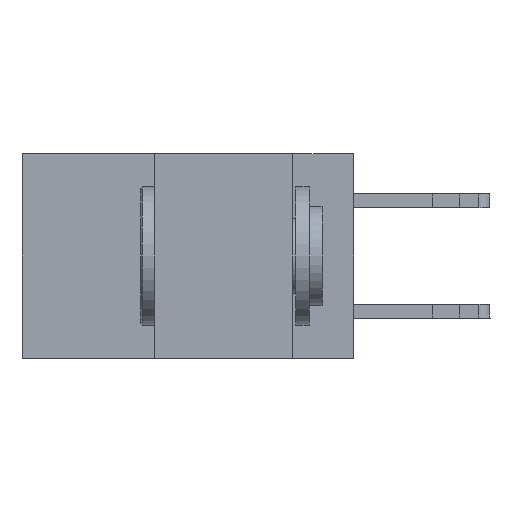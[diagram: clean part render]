
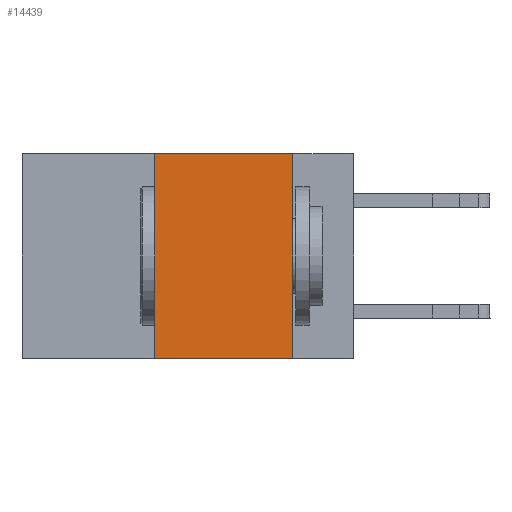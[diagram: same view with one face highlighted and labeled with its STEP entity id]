
A CAD part, left-side view. The second image highlights one B-rep face of the part: STEP entity #14439.
In plain terms, the highlighted planar face has unit normal (-1, 0, 0).
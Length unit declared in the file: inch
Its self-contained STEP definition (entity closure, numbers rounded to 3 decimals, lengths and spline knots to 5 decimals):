
#1233 = DIRECTION ( 'NONE',  ( 0., -1., 0. ) ) ;
#2396 = DIRECTION ( 'NONE',  ( 0., 0., 1. ) ) ;
#2755 = VECTOR ( 'NONE', #1233, 39.37008 ) ;
#3062 = EDGE_LOOP ( 'NONE', ( #3813, #5411, #20418, #20330 ) ) ;
#3558 = EDGE_CURVE ( 'NONE', #17596, #8377, #8873, .T. ) ;
#3753 = VECTOR ( 'NONE', #26122, 39.37008 ) ;
#3813 = ORIENTED_EDGE ( 'NONE', *, *, #18241, .F. ) ;
#4290 = CARTESIAN_POINT ( 'NONE',  ( 0., 0.11, 0. ) ) ;
#4399 = DIRECTION ( 'NONE',  ( 0., 0., -1. ) ) ;
#5411 = ORIENTED_EDGE ( 'NONE', *, *, #3558, .F. ) ;
#8377 = VERTEX_POINT ( 'NONE', #20610 ) ;
#8873 = LINE ( 'NONE', #18444, #3753 ) ;
#9432 = LINE ( 'NONE', #13905, #2755 ) ;
#9440 = FACE_OUTER_BOUND ( 'NONE', #3062, .T. ) ;
#10476 = DIRECTION ( 'NONE',  ( 0., 0., -1. ) ) ;
#10792 = LINE ( 'NONE', #27092, #22492 ) ;
#11726 = LINE ( 'NONE', #4290, #28930 ) ;
#13304 = PLANE ( 'NONE',  #29269 ) ;
#13501 = CARTESIAN_POINT ( 'NONE',  ( 0., 0.36, -0.37 ) ) ;
#13905 = CARTESIAN_POINT ( 'NONE',  ( 0., 0.6, -0.37 ) ) ;
#14439 = ADVANCED_FACE ( 'NONE', ( #9440 ), #13304, .F. ) ;
#15044 = VERTEX_POINT ( 'NONE', #13501 ) ;
#15587 = DIRECTION ( 'NONE',  ( 1., 0., 0. ) ) ;
#17596 = VERTEX_POINT ( 'NONE', #19066 ) ;
#17761 = CARTESIAN_POINT ( 'NONE',  ( 0., 0.11, -0.37 ) ) ;
#18162 = EDGE_CURVE ( 'NONE', #15044, #23795, #9432, .T. ) ;
#18241 = EDGE_CURVE ( 'NONE', #8377, #23795, #11726, .T. ) ;
#18444 = CARTESIAN_POINT ( 'NONE',  ( 0., 0.6, 0. ) ) ;
#19066 = CARTESIAN_POINT ( 'NONE',  ( 0., 0.36, 0. ) ) ;
#20330 = ORIENTED_EDGE ( 'NONE', *, *, #18162, .T. ) ;
#20418 = ORIENTED_EDGE ( 'NONE', *, *, #27899, .F. ) ;
#20610 = CARTESIAN_POINT ( 'NONE',  ( 0., 0.11, 0. ) ) ;
#22492 = VECTOR ( 'NONE', #2396, 39.37008 ) ;
#23008 = CARTESIAN_POINT ( 'NONE',  ( 0., 0.6, 0. ) ) ;
#23795 = VERTEX_POINT ( 'NONE', #17761 ) ;
#26122 = DIRECTION ( 'NONE',  ( 0., -1., 0. ) ) ;
#27092 = CARTESIAN_POINT ( 'NONE',  ( 0., 0.36, 0. ) ) ;
#27899 = EDGE_CURVE ( 'NONE', #15044, #17596, #10792, .T. ) ;
#28930 = VECTOR ( 'NONE', #4399, 39.37008 ) ;
#29269 = AXIS2_PLACEMENT_3D ( 'NONE', #23008, #15587, #10476 ) ;
